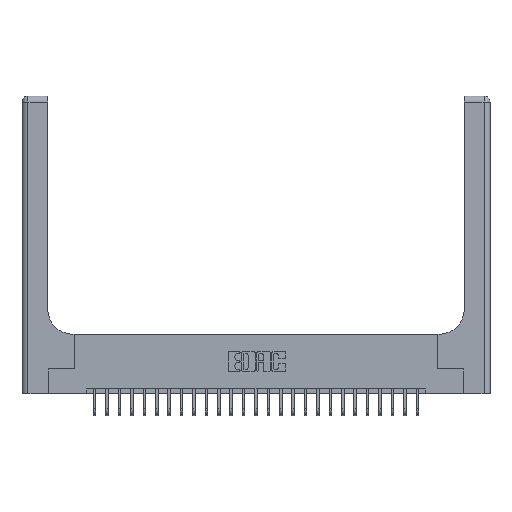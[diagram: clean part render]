
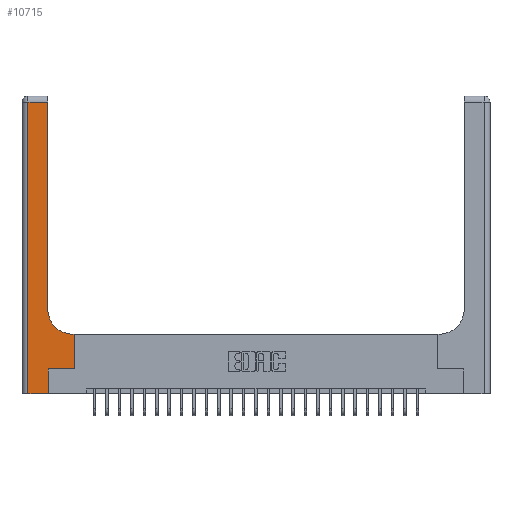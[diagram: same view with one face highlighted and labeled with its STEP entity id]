
A CAD part, top view. The second image highlights one B-rep face of the part: STEP entity #10715.
In plain terms, the highlighted planar face has unit normal (0, 0, 1).
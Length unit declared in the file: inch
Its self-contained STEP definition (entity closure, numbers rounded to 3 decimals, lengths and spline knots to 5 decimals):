
#396 = CARTESIAN_POINT ( 'NONE',  ( 0.26, 2.94, 0.37 ) ) ;
#399 = AXIS2_PLACEMENT_3D ( 'NONE', #8153, #8429, #4596 ) ;
#590 = VERTEX_POINT ( 'NONE', #11225 ) ;
#709 = VECTOR ( 'NONE', #5668, 39.37008 ) ;
#1730 = ORIENTED_EDGE ( 'NONE', *, *, #17346, .T. ) ;
#1733 = CARTESIAN_POINT ( 'NONE',  ( 0.06, 3., 0.37 ) ) ;
#2605 = EDGE_CURVE ( 'NONE', #9777, #12654, #24193, .T. ) ;
#2716 = EDGE_CURVE ( 'NONE', #590, #12729, #17911, .T. ) ;
#3495 = CARTESIAN_POINT ( 'NONE',  ( 0.26, 3., 0.37 ) ) ;
#3862 = VECTOR ( 'NONE', #3919, 39.37008 ) ;
#3919 = DIRECTION ( 'NONE',  ( 0., -1., 0. ) ) ;
#4173 = CARTESIAN_POINT ( 'NONE',  ( 0.528, 0.25, 0.37 ) ) ;
#4596 = DIRECTION ( 'NONE',  ( 1., 0., 0. ) ) ;
#4787 = VECTOR ( 'NONE', #16255, 39.37008 ) ;
#5012 = AXIS2_PLACEMENT_3D ( 'NONE', #24475, #16282, #11763 ) ;
#5542 = EDGE_LOOP ( 'NONE', ( #11187, #18336, #6006, #5716, #25679, #20582, #1730, #12621, #21213 ) ) ;
#5668 = DIRECTION ( 'NONE',  ( 0., 1., 0. ) ) ;
#5716 = ORIENTED_EDGE ( 'NONE', *, *, #24684, .T. ) ;
#6006 = ORIENTED_EDGE ( 'NONE', *, *, #6660, .T. ) ;
#6036 = CARTESIAN_POINT ( 'NONE',  ( 0.265, 0., 0.37 ) ) ;
#6098 = DIRECTION ( 'NONE',  ( 1., 0., 0. ) ) ;
#6107 = VECTOR ( 'NONE', #20580, 39.37008 ) ;
#6660 = EDGE_CURVE ( 'NONE', #25866, #15130, #20495, .T. ) ;
#7057 = LINE ( 'NONE', #15415, #22226 ) ;
#7835 = VECTOR ( 'NONE', #13792, 39.37008 ) ;
#7882 = CARTESIAN_POINT ( 'NONE',  ( 0., 2.94, 0.37 ) ) ;
#8153 = CARTESIAN_POINT ( 'NONE',  ( 0.51, 0.85, 0.37 ) ) ;
#8170 = CARTESIAN_POINT ( 'NONE',  ( 0.06, 2.94, 0.37 ) ) ;
#8390 = EDGE_CURVE ( 'NONE', #12729, #13090, #10045, .T. ) ;
#8429 = DIRECTION ( 'NONE',  ( 0., 0., -1. ) ) ;
#9150 = VERTEX_POINT ( 'NONE', #14968 ) ;
#9366 = DIRECTION ( 'NONE',  ( 0., 1., 0. ) ) ;
#9777 = VERTEX_POINT ( 'NONE', #18289 ) ;
#9824 = FACE_OUTER_BOUND ( 'NONE', #5542, .T. ) ;
#10029 = LINE ( 'NONE', #22618, #22078 ) ;
#10045 = LINE ( 'NONE', #3495, #709 ) ;
#10078 = CARTESIAN_POINT ( 'NONE',  ( 0.265, 0.25, 0.37 ) ) ;
#10486 = CARTESIAN_POINT ( 'NONE',  ( 0., 0., 0.37 ) ) ;
#10715 = ADVANCED_FACE ( 'NONE', ( #9824 ), #11899, .F. ) ;
#11187 = ORIENTED_EDGE ( 'NONE', *, *, #8390, .T. ) ;
#11225 = CARTESIAN_POINT ( 'NONE',  ( 0.51, 0.6, 0.37 ) ) ;
#11246 = EDGE_CURVE ( 'NONE', #9150, #590, #10029, .T. ) ;
#11763 = DIRECTION ( 'NONE',  ( -1., 0., 0. ) ) ;
#11899 = PLANE ( 'NONE',  #5012 ) ;
#12421 = LINE ( 'NONE', #10486, #24904 ) ;
#12621 = ORIENTED_EDGE ( 'NONE', *, *, #11246, .T. ) ;
#12654 = VERTEX_POINT ( 'NONE', #4173 ) ;
#12729 = VERTEX_POINT ( 'NONE', #25940 ) ;
#13090 = VERTEX_POINT ( 'NONE', #396 ) ;
#13792 = DIRECTION ( 'NONE',  ( 1., 0., 0. ) ) ;
#14968 = CARTESIAN_POINT ( 'NONE',  ( 0.528, 0.6, 0.37 ) ) ;
#15119 = CARTESIAN_POINT ( 'NONE',  ( 0.265, 0., 0.37 ) ) ;
#15130 = VERTEX_POINT ( 'NONE', #17268 ) ;
#15415 = CARTESIAN_POINT ( 'NONE',  ( 0.528, 0.25, 0.37 ) ) ;
#16255 = DIRECTION ( 'NONE',  ( -1., 0., 0. ) ) ;
#16282 = DIRECTION ( 'NONE',  ( 0., 0., -1. ) ) ;
#16481 = DIRECTION ( 'NONE',  ( -1., 0., 0. ) ) ;
#17268 = CARTESIAN_POINT ( 'NONE',  ( 0.06, 0., 0.37 ) ) ;
#17346 = EDGE_CURVE ( 'NONE', #12654, #9150, #7057, .T. ) ;
#17911 = CIRCLE ( 'NONE', #399, 0.25 ) ;
#18263 = LINE ( 'NONE', #6036, #6107 ) ;
#18289 = CARTESIAN_POINT ( 'NONE',  ( 0.265, 0.25, 0.37 ) ) ;
#18336 = ORIENTED_EDGE ( 'NONE', *, *, #18912, .T. ) ;
#18912 = EDGE_CURVE ( 'NONE', #13090, #25866, #26646, .T. ) ;
#20495 = LINE ( 'NONE', #1733, #3862 ) ;
#20580 = DIRECTION ( 'NONE',  ( 0., 1., 0. ) ) ;
#20582 = ORIENTED_EDGE ( 'NONE', *, *, #2605, .T. ) ;
#20931 = VERTEX_POINT ( 'NONE', #15119 ) ;
#21213 = ORIENTED_EDGE ( 'NONE', *, *, #2716, .T. ) ;
#22078 = VECTOR ( 'NONE', #16481, 39.37008 ) ;
#22226 = VECTOR ( 'NONE', #9366, 39.37008 ) ;
#22618 = CARTESIAN_POINT ( 'NONE',  ( 0.26, 0.6, 0.37 ) ) ;
#24193 = LINE ( 'NONE', #10078, #7835 ) ;
#24475 = CARTESIAN_POINT ( 'NONE',  ( 0., 3., 0.37 ) ) ;
#24684 = EDGE_CURVE ( 'NONE', #15130, #20931, #12421, .T. ) ;
#24904 = VECTOR ( 'NONE', #6098, 39.37008 ) ;
#25540 = EDGE_CURVE ( 'NONE', #20931, #9777, #18263, .T. ) ;
#25679 = ORIENTED_EDGE ( 'NONE', *, *, #25540, .T. ) ;
#25866 = VERTEX_POINT ( 'NONE', #8170 ) ;
#25940 = CARTESIAN_POINT ( 'NONE',  ( 0.26, 0.85, 0.37 ) ) ;
#26646 = LINE ( 'NONE', #7882, #4787 ) ;
